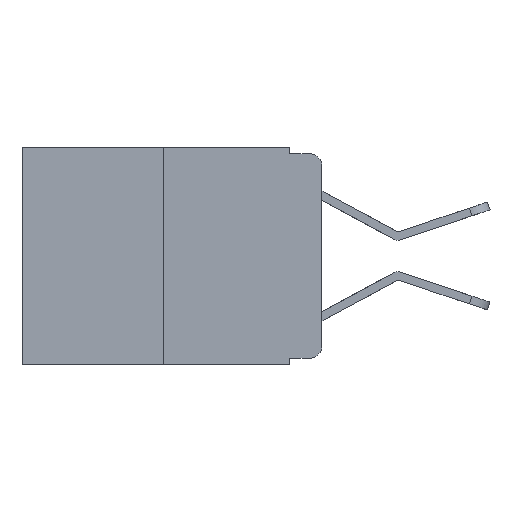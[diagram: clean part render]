
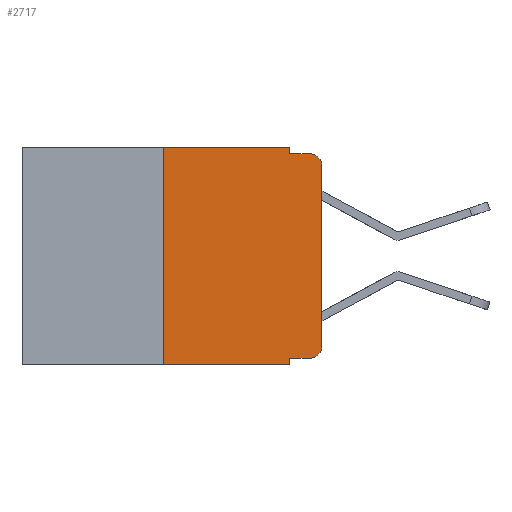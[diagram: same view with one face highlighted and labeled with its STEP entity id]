
A CAD part, left-side view. The second image highlights one B-rep face of the part: STEP entity #2717.
In plain terms, the highlighted planar face has unit normal (-1, 0, 0).
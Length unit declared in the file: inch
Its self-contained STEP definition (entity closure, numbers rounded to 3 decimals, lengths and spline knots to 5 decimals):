
#255 = DIRECTION ( 'NONE',  ( -1., 0., 0. ) ) ;
#287 = DIRECTION ( 'NONE',  ( 0., 0., -1. ) ) ;
#445 = ORIENTED_EDGE ( 'NONE', *, *, #1480, .T. ) ;
#705 = PLANE ( 'NONE',  #11989 ) ;
#943 = LINE ( 'NONE', #7155, #10678 ) ;
#990 = LINE ( 'NONE', #9783, #3748 ) ;
#1035 = CARTESIAN_POINT ( 'NONE',  ( 0., 0.051, -0.01 ) ) ;
#1234 = CARTESIAN_POINT ( 'NONE',  ( 0., 0.473, 0. ) ) ;
#1302 = VERTEX_POINT ( 'NONE', #1345 ) ;
#1303 = CARTESIAN_POINT ( 'NONE',  ( 0., 0.051, -0.01 ) ) ;
#1345 = CARTESIAN_POINT ( 'NONE',  ( 0., 0.25, -0.343 ) ) ;
#1397 = DIRECTION ( 'NONE',  ( -1., 0., 0. ) ) ;
#1431 = CARTESIAN_POINT ( 'NONE',  ( 0., 0.02, -0.03 ) ) ;
#1480 = EDGE_CURVE ( 'NONE', #1302, #11548, #2901, .T. ) ;
#1626 = DIRECTION ( 'NONE',  ( 0., -1., 0. ) ) ;
#1642 = CARTESIAN_POINT ( 'NONE',  ( 0., 0.473, 0. ) ) ;
#1739 = VECTOR ( 'NONE', #1626, 39.37008 ) ;
#1843 = CARTESIAN_POINT ( 'NONE',  ( 0., 0.051, 0. ) ) ;
#1972 = EDGE_CURVE ( 'NONE', #10865, #11091, #5444, .T. ) ;
#1983 = DIRECTION ( 'NONE',  ( 0., -1., 0. ) ) ;
#2259 = LINE ( 'NONE', #1035, #11740 ) ;
#2275 = ORIENTED_EDGE ( 'NONE', *, *, #6834, .F. ) ;
#2519 = VERTEX_POINT ( 'NONE', #7074 ) ;
#2610 = ORIENTED_EDGE ( 'NONE', *, *, #5837, .T. ) ;
#2717 = ADVANCED_FACE ( 'NONE', ( #11721 ), #705, .F. ) ;
#2901 = LINE ( 'NONE', #10639, #11973 ) ;
#3367 = CARTESIAN_POINT ( 'NONE',  ( 0., 0.051, -0.343 ) ) ;
#3390 = DIRECTION ( 'NONE',  ( 0., 0., -1. ) ) ;
#3586 = ORIENTED_EDGE ( 'NONE', *, *, #6305, .F. ) ;
#3604 = DIRECTION ( 'NONE',  ( 0., 0., -1. ) ) ;
#3748 = VECTOR ( 'NONE', #3390, 39.37008 ) ;
#4010 = EDGE_CURVE ( 'NONE', #10865, #11548, #9636, .T. ) ;
#4189 = VERTEX_POINT ( 'NONE', #9295 ) ;
#4363 = CIRCLE ( 'NONE', #4959, 0.02 ) ;
#4877 = ORIENTED_EDGE ( 'NONE', *, *, #5599, .F. ) ;
#4880 = DIRECTION ( 'NONE',  ( 0., 0., 1. ) ) ;
#4959 = AXIS2_PLACEMENT_3D ( 'NONE', #7199, #1397, #3604 ) ;
#5040 = CARTESIAN_POINT ( 'NONE',  ( 0., 0., -0.313 ) ) ;
#5249 = EDGE_CURVE ( 'NONE', #8647, #2519, #943, .T. ) ;
#5444 = LINE ( 'NONE', #9971, #9664 ) ;
#5599 = EDGE_CURVE ( 'NONE', #7389, #4189, #2259, .T. ) ;
#5837 = EDGE_CURVE ( 'NONE', #2519, #4189, #11597, .T. ) ;
#6015 = LINE ( 'NONE', #11809, #8170 ) ;
#6063 = DIRECTION ( 'NONE',  ( 0., 0., 1. ) ) ;
#6305 = EDGE_CURVE ( 'NONE', #8373, #11115, #6894, .T. ) ;
#6362 = ORIENTED_EDGE ( 'NONE', *, *, #9116, .T. ) ;
#6834 = EDGE_CURVE ( 'NONE', #1302, #8373, #6015, .T. ) ;
#6894 = LINE ( 'NONE', #1642, #1739 ) ;
#7074 = CARTESIAN_POINT ( 'NONE',  ( 0., 0., -0.03 ) ) ;
#7155 = CARTESIAN_POINT ( 'NONE',  ( 0., 0., 0. ) ) ;
#7199 = CARTESIAN_POINT ( 'NONE',  ( 0., 0.02, -0.313 ) ) ;
#7389 = VERTEX_POINT ( 'NONE', #1303 ) ;
#7582 = DIRECTION ( 'NONE',  ( 0., -1., 0. ) ) ;
#7667 = CARTESIAN_POINT ( 'NONE',  ( 0., 0.051, 0. ) ) ;
#8166 = DIRECTION ( 'NONE',  ( 1., 0., 0. ) ) ;
#8170 = VECTOR ( 'NONE', #6063, 39.37008 ) ;
#8208 = ORIENTED_EDGE ( 'NONE', *, *, #12139, .F. ) ;
#8333 = DIRECTION ( 'NONE',  ( 0., -1., 0. ) ) ;
#8373 = VERTEX_POINT ( 'NONE', #10406 ) ;
#8647 = VERTEX_POINT ( 'NONE', #5040 ) ;
#8767 = ORIENTED_EDGE ( 'NONE', *, *, #1972, .T. ) ;
#9116 = EDGE_CURVE ( 'NONE', #11091, #8647, #4363, .T. ) ;
#9295 = CARTESIAN_POINT ( 'NONE',  ( 0., 0.02, -0.01 ) ) ;
#9636 = LINE ( 'NONE', #1843, #12208 ) ;
#9664 = VECTOR ( 'NONE', #8333, 39.37008 ) ;
#9715 = ORIENTED_EDGE ( 'NONE', *, *, #4010, .F. ) ;
#9783 = CARTESIAN_POINT ( 'NONE',  ( 0., 0.051, 0. ) ) ;
#9936 = DIRECTION ( 'NONE',  ( 0., 0., -1. ) ) ;
#9971 = CARTESIAN_POINT ( 'NONE',  ( 0., 0.051, -0.333 ) ) ;
#9982 = EDGE_LOOP ( 'NONE', ( #11351, #2610, #4877, #8208, #3586, #2275, #445, #9715, #8767, #6362 ) ) ;
#10406 = CARTESIAN_POINT ( 'NONE',  ( 0., 0.25, 0. ) ) ;
#10639 = CARTESIAN_POINT ( 'NONE',  ( 0., 0.473, -0.343 ) ) ;
#10678 = VECTOR ( 'NONE', #4880, 39.37008 ) ;
#10865 = VERTEX_POINT ( 'NONE', #11093 ) ;
#11018 = AXIS2_PLACEMENT_3D ( 'NONE', #1431, #255, #287 ) ;
#11091 = VERTEX_POINT ( 'NONE', #12017 ) ;
#11093 = CARTESIAN_POINT ( 'NONE',  ( 0., 0.051, -0.333 ) ) ;
#11115 = VERTEX_POINT ( 'NONE', #7667 ) ;
#11351 = ORIENTED_EDGE ( 'NONE', *, *, #5249, .T. ) ;
#11461 = DIRECTION ( 'NONE',  ( 0., 0., -1. ) ) ;
#11548 = VERTEX_POINT ( 'NONE', #3367 ) ;
#11597 = CIRCLE ( 'NONE', #11018, 0.02 ) ;
#11721 = FACE_OUTER_BOUND ( 'NONE', #9982, .T. ) ;
#11740 = VECTOR ( 'NONE', #7582, 39.37008 ) ;
#11809 = CARTESIAN_POINT ( 'NONE',  ( 0., 0.25, 0. ) ) ;
#11973 = VECTOR ( 'NONE', #1983, 39.37008 ) ;
#11989 = AXIS2_PLACEMENT_3D ( 'NONE', #1234, #8166, #11461 ) ;
#12017 = CARTESIAN_POINT ( 'NONE',  ( 0., 0.02, -0.333 ) ) ;
#12139 = EDGE_CURVE ( 'NONE', #11115, #7389, #990, .T. ) ;
#12208 = VECTOR ( 'NONE', #9936, 39.37008 ) ;
